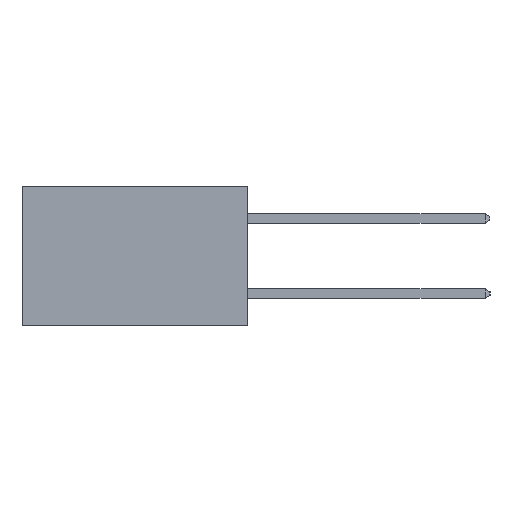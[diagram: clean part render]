
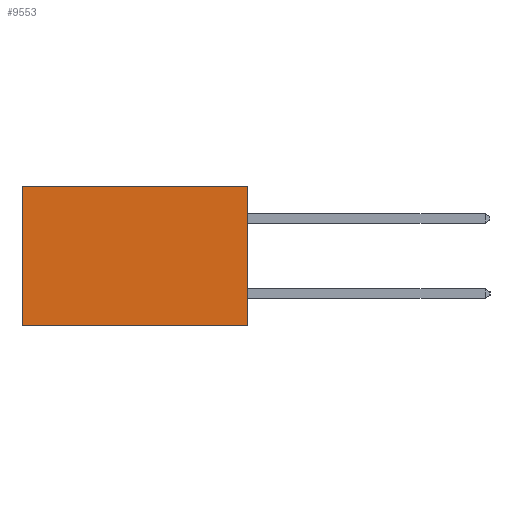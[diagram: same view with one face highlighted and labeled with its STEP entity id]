
A CAD part, left-side view. The second image highlights one B-rep face of the part: STEP entity #9553.
In plain terms, the highlighted planar face has unit normal (-1, 0, 0).
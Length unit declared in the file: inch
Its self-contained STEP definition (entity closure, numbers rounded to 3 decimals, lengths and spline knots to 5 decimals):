
#378 = CARTESIAN_POINT ( 'NONE',  ( 0.2615, 0.6, -0.37 ) ) ;
#665 = LINE ( 'NONE', #378, #11267 ) ;
#963 = DIRECTION ( 'NONE',  ( 0., 0., -1. ) ) ;
#1496 = CARTESIAN_POINT ( 'NONE',  ( 0.2615, 0., 0. ) ) ;
#1920 = ORIENTED_EDGE ( 'NONE', *, *, #6851, .F. ) ;
#1947 = EDGE_CURVE ( 'NONE', #5277, #12459, #665, .T. ) ;
#1956 = CARTESIAN_POINT ( 'NONE',  ( 0.2615, 0., 0. ) ) ;
#2133 = FACE_OUTER_BOUND ( 'NONE', #13598, .T. ) ;
#2147 = EDGE_CURVE ( 'NONE', #15832, #11746, #13622, .T. ) ;
#2295 = PLANE ( 'NONE',  #10760 ) ;
#3273 = LINE ( 'NONE', #4035, #7411 ) ;
#3442 = ORIENTED_EDGE ( 'NONE', *, *, #14934, .T. ) ;
#4035 = CARTESIAN_POINT ( 'NONE',  ( 0.2615, 0., -0.37 ) ) ;
#5233 = DIRECTION ( 'NONE',  ( 0., 0., -1. ) ) ;
#5277 = VERTEX_POINT ( 'NONE', #7930 ) ;
#5760 = DIRECTION ( 'NONE',  ( 0., 0., -1. ) ) ;
#6426 = ORIENTED_EDGE ( 'NONE', *, *, #2147, .F. ) ;
#6457 = VECTOR ( 'NONE', #5760, 39.37008 ) ;
#6851 = EDGE_CURVE ( 'NONE', #11746, #12459, #3273, .T. ) ;
#7411 = VECTOR ( 'NONE', #13555, 39.37008 ) ;
#7745 = CARTESIAN_POINT ( 'NONE',  ( 0.2615, 0.6, -0.37 ) ) ;
#7930 = CARTESIAN_POINT ( 'NONE',  ( 0.2615, 0.6, 0. ) ) ;
#9035 = CARTESIAN_POINT ( 'NONE',  ( 0.2615, 0., -0.37 ) ) ;
#9292 = DIRECTION ( 'NONE',  ( 1., 0., 0. ) ) ;
#9553 = ADVANCED_FACE ( 'NONE', ( #2133 ), #2295, .F. ) ;
#10760 = AXIS2_PLACEMENT_3D ( 'NONE', #14551, #9292, #963 ) ;
#11267 = VECTOR ( 'NONE', #5233, 39.37008 ) ;
#11746 = VERTEX_POINT ( 'NONE', #9035 ) ;
#12459 = VERTEX_POINT ( 'NONE', #7745 ) ;
#13555 = DIRECTION ( 'NONE',  ( 0., 1., 0. ) ) ;
#13598 = EDGE_LOOP ( 'NONE', ( #15225, #1920, #6426, #3442 ) ) ;
#13622 = LINE ( 'NONE', #16483, #6457 ) ;
#13661 = VECTOR ( 'NONE', #15107, 39.37008 ) ;
#14082 = LINE ( 'NONE', #1496, #13661 ) ;
#14551 = CARTESIAN_POINT ( 'NONE',  ( 0.2615, 0., -0.37 ) ) ;
#14934 = EDGE_CURVE ( 'NONE', #15832, #5277, #14082, .T. ) ;
#15107 = DIRECTION ( 'NONE',  ( 0., 1., 0. ) ) ;
#15225 = ORIENTED_EDGE ( 'NONE', *, *, #1947, .T. ) ;
#15832 = VERTEX_POINT ( 'NONE', #1956 ) ;
#16483 = CARTESIAN_POINT ( 'NONE',  ( 0.2615, 0., -0.37 ) ) ;
